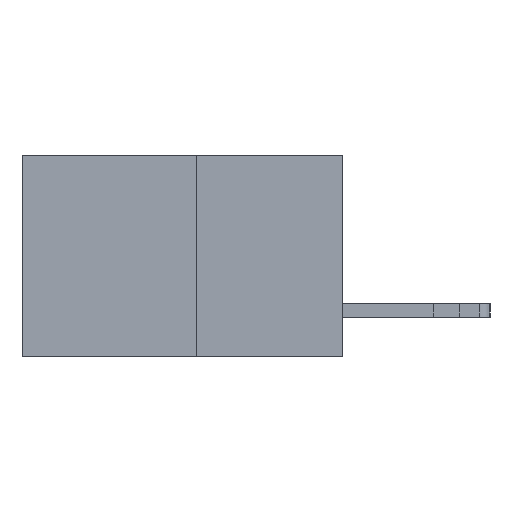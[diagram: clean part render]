
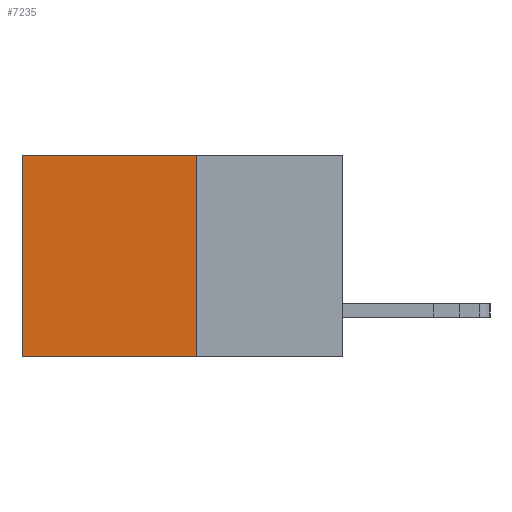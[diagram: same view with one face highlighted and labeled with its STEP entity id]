
A CAD part, left-side view. The second image highlights one B-rep face of the part: STEP entity #7235.
In plain terms, the highlighted planar face has unit normal (-1, 0, 0).
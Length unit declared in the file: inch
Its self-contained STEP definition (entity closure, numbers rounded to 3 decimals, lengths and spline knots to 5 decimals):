
#222 = CARTESIAN_POINT ( 'NONE',  ( 0.277, 0.27, 0. ) ) ;
#669 = CARTESIAN_POINT ( 'NONE',  ( 0.277, 0.27, -0.37 ) ) ;
#1903 = CARTESIAN_POINT ( 'NONE',  ( 0.277, 0.27, -0.37 ) ) ;
#2212 = FACE_OUTER_BOUND ( 'NONE', #14464, .T. ) ;
#2262 = ORIENTED_EDGE ( 'NONE', *, *, #16739, .F. ) ;
#2804 = EDGE_CURVE ( 'NONE', #5462, #16028, #17992, .T. ) ;
#3553 = PLANE ( 'NONE',  #12859 ) ;
#3785 = LINE ( 'NONE', #669, #7063 ) ;
#5188 = DIRECTION ( 'NONE',  ( 1., 0., 0. ) ) ;
#5462 = VERTEX_POINT ( 'NONE', #16553 ) ;
#6119 = EDGE_CURVE ( 'NONE', #18847, #16028, #3785, .T. ) ;
#6649 = VECTOR ( 'NONE', #17584, 39.37008 ) ;
#6944 = EDGE_CURVE ( 'NONE', #7892, #5462, #12619, .T. ) ;
#7063 = VECTOR ( 'NONE', #7205, 39.37008 ) ;
#7205 = DIRECTION ( 'NONE',  ( 0., 1., 0. ) ) ;
#7235 = ADVANCED_FACE ( 'NONE', ( #2212 ), #3553, .F. ) ;
#7892 = VERTEX_POINT ( 'NONE', #222 ) ;
#8931 = ORIENTED_EDGE ( 'NONE', *, *, #6119, .F. ) ;
#9262 = DIRECTION ( 'NONE',  ( 0., 1., 0. ) ) ;
#11689 = ORIENTED_EDGE ( 'NONE', *, *, #2804, .T. ) ;
#12619 = LINE ( 'NONE', #17280, #20617 ) ;
#12859 = AXIS2_PLACEMENT_3D ( 'NONE', #1903, #5188, #16424 ) ;
#14464 = EDGE_LOOP ( 'NONE', ( #11689, #8931, #2262, #16640 ) ) ;
#14768 = DIRECTION ( 'NONE',  ( 0., 0., -1. ) ) ;
#15994 = CARTESIAN_POINT ( 'NONE',  ( 0.277, 0.27, -0.37 ) ) ;
#16028 = VERTEX_POINT ( 'NONE', #20336 ) ;
#16424 = DIRECTION ( 'NONE',  ( 0., 0., -1. ) ) ;
#16553 = CARTESIAN_POINT ( 'NONE',  ( 0.277, 0.59, 0. ) ) ;
#16640 = ORIENTED_EDGE ( 'NONE', *, *, #6944, .T. ) ;
#16739 = EDGE_CURVE ( 'NONE', #7892, #18847, #18932, .T. ) ;
#16969 = CARTESIAN_POINT ( 'NONE',  ( 0.277, 0.27, -0.37 ) ) ;
#17280 = CARTESIAN_POINT ( 'NONE',  ( 0.277, 0.27, 0. ) ) ;
#17519 = VECTOR ( 'NONE', #14768, 39.37008 ) ;
#17584 = DIRECTION ( 'NONE',  ( 0., 0., -1. ) ) ;
#17623 = CARTESIAN_POINT ( 'NONE',  ( 0.277, 0.59, -0.37 ) ) ;
#17992 = LINE ( 'NONE', #17623, #17519 ) ;
#18847 = VERTEX_POINT ( 'NONE', #16969 ) ;
#18932 = LINE ( 'NONE', #15994, #6649 ) ;
#20336 = CARTESIAN_POINT ( 'NONE',  ( 0.277, 0.59, -0.37 ) ) ;
#20617 = VECTOR ( 'NONE', #9262, 39.37008 ) ;
